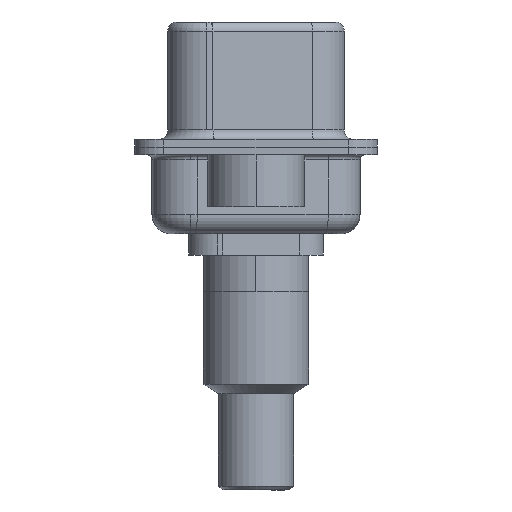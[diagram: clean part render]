
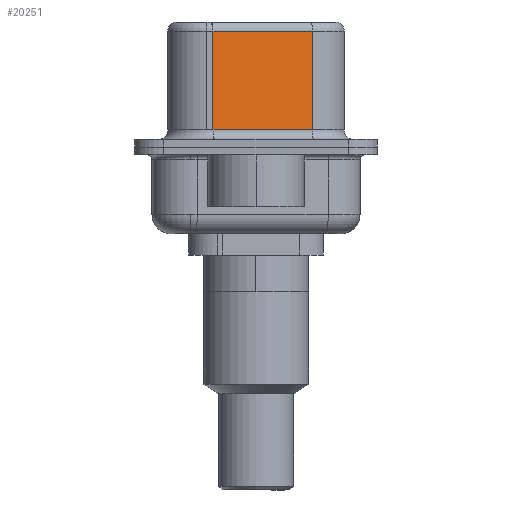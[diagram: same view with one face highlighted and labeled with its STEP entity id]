
A CAD part, left-side view. The second image highlights one B-rep face of the part: STEP entity #20251.
In plain terms, the highlighted planar face has unit normal (-0.985, -0.174, 0).
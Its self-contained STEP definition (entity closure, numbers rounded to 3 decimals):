
#169 = CARTESIAN_POINT ( 'NONE',  ( 4.58, -2.927, 6.02 ) ) ;
#1109 = ORIENTED_EDGE ( 'NONE', *, *, #20440, .T. ) ;
#1959 = AXIS2_PLACEMENT_3D ( 'NONE', #28804, #28921, #15459 ) ;
#2387 = CARTESIAN_POINT ( 'NONE',  ( 4.58, -2.927, 0.9 ) ) ;
#2635 = VERTEX_POINT ( 'NONE', #14810 ) ;
#4937 = ORIENTED_EDGE ( 'NONE', *, *, #16471, .T. ) ;
#6009 = LINE ( 'NONE', #169, #22689 ) ;
#8590 = PLANE ( 'NONE',  #1959 ) ;
#10407 = CARTESIAN_POINT ( 'NONE',  ( 4.58, -2.927, 6.52 ) ) ;
#10810 = CARTESIAN_POINT ( 'NONE',  ( 4.58, -2.927, 0.9 ) ) ;
#11674 = LINE ( 'NONE', #19528, #16955 ) ;
#11740 = DIRECTION ( 'NONE',  ( -0.174, 0.985, 0. ) ) ;
#12398 = ORIENTED_EDGE ( 'NONE', *, *, #26435, .T. ) ;
#14090 = VERTEX_POINT ( 'NONE', #10810 ) ;
#14810 = CARTESIAN_POINT ( 'NONE',  ( 4.58, -2.927, 6.02 ) ) ;
#15459 = DIRECTION ( 'NONE',  ( -0.174, 0.985, 0. ) ) ;
#15860 = LINE ( 'NONE', #2387, #21165 ) ;
#16471 = EDGE_CURVE ( 'NONE', #21894, #23695, #11674, .T. ) ;
#16955 = VECTOR ( 'NONE', #17279, 1000. ) ;
#17135 = DIRECTION ( 'NONE',  ( 0., 0., -1. ) ) ;
#17279 = DIRECTION ( 'NONE',  ( 0., 0., -1. ) ) ;
#18760 = LINE ( 'NONE', #10407, #28562 ) ;
#19356 = EDGE_LOOP ( 'NONE', ( #22670, #12398, #4937, #1109 ) ) ;
#19528 = CARTESIAN_POINT ( 'NONE',  ( 3.67, 2.233, 6.52 ) ) ;
#20251 = ADVANCED_FACE ( 'NONE', ( #26048 ), #8590, .F. ) ;
#20440 = EDGE_CURVE ( 'NONE', #23695, #14090, #15860, .T. ) ;
#21165 = VECTOR ( 'NONE', #25076, 1000. ) ;
#21469 = CARTESIAN_POINT ( 'NONE',  ( 3.67, 2.233, 0.9 ) ) ;
#21894 = VERTEX_POINT ( 'NONE', #27577 ) ;
#22670 = ORIENTED_EDGE ( 'NONE', *, *, #27574, .F. ) ;
#22689 = VECTOR ( 'NONE', #11740, 1000. ) ;
#23695 = VERTEX_POINT ( 'NONE', #21469 ) ;
#25076 = DIRECTION ( 'NONE',  ( 0.174, -0.985, 0. ) ) ;
#26048 = FACE_OUTER_BOUND ( 'NONE', #19356, .T. ) ;
#26435 = EDGE_CURVE ( 'NONE', #2635, #21894, #6009, .T. ) ;
#27574 = EDGE_CURVE ( 'NONE', #2635, #14090, #18760, .T. ) ;
#27577 = CARTESIAN_POINT ( 'NONE',  ( 3.67, 2.233, 6.02 ) ) ;
#28562 = VECTOR ( 'NONE', #17135, 1000. ) ;
#28804 = CARTESIAN_POINT ( 'NONE',  ( 4.58, -2.927, 6.52 ) ) ;
#28921 = DIRECTION ( 'NONE',  ( 0.985, 0.174, 0. ) ) ;
